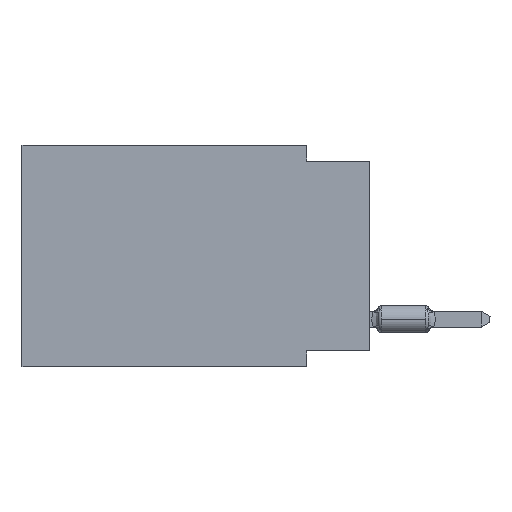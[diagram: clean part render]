
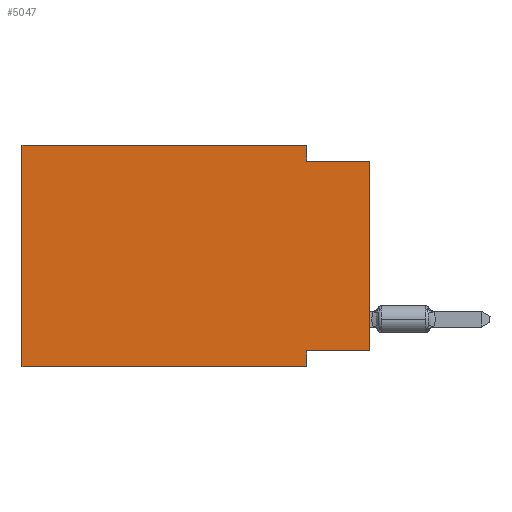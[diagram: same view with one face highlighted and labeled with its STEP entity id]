
A CAD part, left-side view. The second image highlights one B-rep face of the part: STEP entity #5047.
In plain terms, the highlighted planar face has unit normal (-1, 0, 0).
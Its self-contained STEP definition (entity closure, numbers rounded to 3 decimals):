
#635 = CARTESIAN_POINT ( 'NONE',  ( 0., 0., -8.255 ) ) ;
#1150 = CARTESIAN_POINT ( 'NONE',  ( 0., 0., -0.635 ) ) ;
#1504 = VERTEX_POINT ( 'NONE', #1150 ) ;
#1943 = PLANE ( 'NONE',  #23656 ) ;
#3065 = VECTOR ( 'NONE', #24060, 1000. ) ;
#3158 = DIRECTION ( 'NONE',  ( 1., 0., 0. ) ) ;
#3901 = VERTEX_POINT ( 'NONE', #25355 ) ;
#3904 = DIRECTION ( 'NONE',  ( 0., -1., 0. ) ) ;
#4154 = ORIENTED_EDGE ( 'NONE', *, *, #9433, .F. ) ;
#4666 = FACE_OUTER_BOUND ( 'NONE', #21447, .T. ) ;
#5002 = VECTOR ( 'NONE', #3904, 1000. ) ;
#5047 = ADVANCED_FACE ( 'NONE', ( #4666 ), #1943, .F. ) ;
#5048 = CARTESIAN_POINT ( 'NONE',  ( 0., 13.97, -8.89 ) ) ;
#5141 = VECTOR ( 'NONE', #11425, 1000. ) ;
#5369 = CARTESIAN_POINT ( 'NONE',  ( 0., 0., -8.255 ) ) ;
#5403 = VERTEX_POINT ( 'NONE', #20858 ) ;
#5555 = CARTESIAN_POINT ( 'NONE',  ( 0., 0., 0. ) ) ;
#5880 = EDGE_CURVE ( 'NONE', #13218, #7715, #7491, .T. ) ;
#7184 = VECTOR ( 'NONE', #21920, 1000. ) ;
#7322 = ORIENTED_EDGE ( 'NONE', *, *, #15906, .F. ) ;
#7491 = LINE ( 'NONE', #5048, #7184 ) ;
#7550 = ORIENTED_EDGE ( 'NONE', *, *, #20770, .F. ) ;
#7715 = VERTEX_POINT ( 'NONE', #12099 ) ;
#7734 = DIRECTION ( 'NONE',  ( 0., 0., -1. ) ) ;
#8153 = VECTOR ( 'NONE', #15849, 1000. ) ;
#8545 = LINE ( 'NONE', #635, #21910 ) ;
#8604 = CARTESIAN_POINT ( 'NONE',  ( 0., 2.54, -8.255 ) ) ;
#8704 = EDGE_CURVE ( 'NONE', #13218, #3901, #9118, .T. ) ;
#8902 = DIRECTION ( 'NONE',  ( 0., 0., -1. ) ) ;
#9118 = LINE ( 'NONE', #17431, #9858 ) ;
#9166 = ORIENTED_EDGE ( 'NONE', *, *, #5880, .T. ) ;
#9433 = EDGE_CURVE ( 'NONE', #14975, #5403, #21824, .T. ) ;
#9646 = DIRECTION ( 'NONE',  ( 0., 0., 1. ) ) ;
#9858 = VECTOR ( 'NONE', #9646, 1000. ) ;
#9911 = LINE ( 'NONE', #26641, #26291 ) ;
#10260 = CARTESIAN_POINT ( 'NONE',  ( 0., 13.97, 0. ) ) ;
#10710 = CARTESIAN_POINT ( 'NONE',  ( 0., 2.54, 0. ) ) ;
#11411 = EDGE_CURVE ( 'NONE', #18758, #1504, #19873, .T. ) ;
#11425 = DIRECTION ( 'NONE',  ( 0., 0., 1. ) ) ;
#12099 = CARTESIAN_POINT ( 'NONE',  ( 0., 2.54, -8.89 ) ) ;
#13142 = ORIENTED_EDGE ( 'NONE', *, *, #8704, .F. ) ;
#13218 = VERTEX_POINT ( 'NONE', #26390 ) ;
#14076 = ORIENTED_EDGE ( 'NONE', *, *, #19516, .F. ) ;
#14975 = VERTEX_POINT ( 'NONE', #10710 ) ;
#15343 = VERTEX_POINT ( 'NONE', #8604 ) ;
#15741 = ORIENTED_EDGE ( 'NONE', *, *, #11411, .T. ) ;
#15849 = DIRECTION ( 'NONE',  ( 0., 0., -1. ) ) ;
#15906 = EDGE_CURVE ( 'NONE', #3901, #14975, #19335, .T. ) ;
#17265 = DIRECTION ( 'NONE',  ( 0., 1., 0. ) ) ;
#17431 = CARTESIAN_POINT ( 'NONE',  ( 0., 13.97, 0. ) ) ;
#18226 = CARTESIAN_POINT ( 'NONE',  ( 0., 0., -0.635 ) ) ;
#18758 = VERTEX_POINT ( 'NONE', #5369 ) ;
#19335 = LINE ( 'NONE', #21755, #3065 ) ;
#19516 = EDGE_CURVE ( 'NONE', #18758, #15343, #8545, .T. ) ;
#19802 = CARTESIAN_POINT ( 'NONE',  ( 0., 2.54, 0. ) ) ;
#19873 = LINE ( 'NONE', #5555, #5141 ) ;
#20729 = EDGE_CURVE ( 'NONE', #15343, #7715, #9911, .T. ) ;
#20770 = EDGE_CURVE ( 'NONE', #5403, #1504, #22418, .T. ) ;
#20858 = CARTESIAN_POINT ( 'NONE',  ( 0., 2.54, -0.635 ) ) ;
#21447 = EDGE_LOOP ( 'NONE', ( #15741, #7550, #4154, #7322, #13142, #9166, #25895, #14076 ) ) ;
#21755 = CARTESIAN_POINT ( 'NONE',  ( 0., 13.97, 0. ) ) ;
#21824 = LINE ( 'NONE', #19802, #8153 ) ;
#21910 = VECTOR ( 'NONE', #17265, 1000. ) ;
#21920 = DIRECTION ( 'NONE',  ( 0., -1., 0. ) ) ;
#22418 = LINE ( 'NONE', #18226, #5002 ) ;
#23656 = AXIS2_PLACEMENT_3D ( 'NONE', #10260, #3158, #8902 ) ;
#24060 = DIRECTION ( 'NONE',  ( 0., -1., 0. ) ) ;
#25355 = CARTESIAN_POINT ( 'NONE',  ( 0., 13.97, 0. ) ) ;
#25895 = ORIENTED_EDGE ( 'NONE', *, *, #20729, .F. ) ;
#26291 = VECTOR ( 'NONE', #7734, 1000. ) ;
#26390 = CARTESIAN_POINT ( 'NONE',  ( 0., 13.97, -8.89 ) ) ;
#26641 = CARTESIAN_POINT ( 'NONE',  ( 0., 2.54, -8.89 ) ) ;
